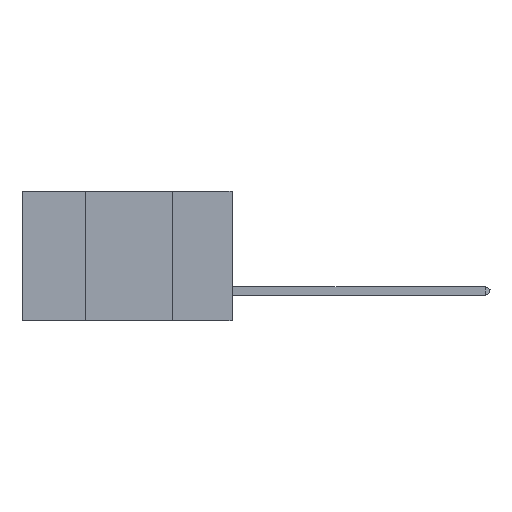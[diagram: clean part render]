
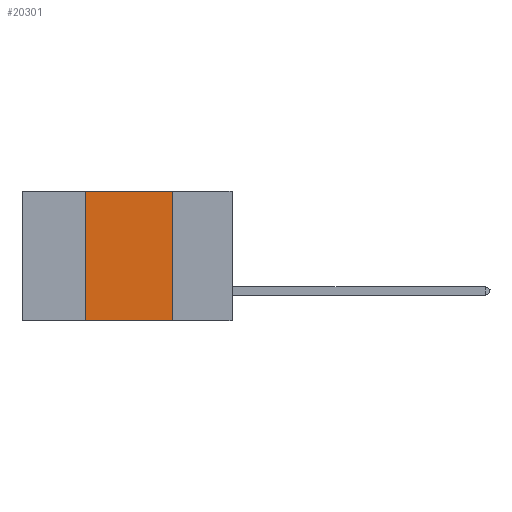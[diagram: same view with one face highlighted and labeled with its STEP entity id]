
A CAD part, left-side view. The second image highlights one B-rep face of the part: STEP entity #20301.
In plain terms, the highlighted planar face has unit normal (-1, 0, 0).
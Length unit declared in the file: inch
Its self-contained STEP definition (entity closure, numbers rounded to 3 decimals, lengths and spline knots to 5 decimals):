
#826 = VERTEX_POINT ( 'NONE', #9016 ) ;
#1259 = DIRECTION ( 'NONE',  ( 0., -1., 0. ) ) ;
#1552 = VECTOR ( 'NONE', #9663, 39.37008 ) ;
#1817 = LINE ( 'NONE', #21628, #24952 ) ;
#1890 = DIRECTION ( 'NONE',  ( 1., 0., 0. ) ) ;
#2437 = EDGE_CURVE ( 'NONE', #2929, #826, #20602, .T. ) ;
#2929 = VERTEX_POINT ( 'NONE', #21281 ) ;
#3544 = CARTESIAN_POINT ( 'NONE',  ( 0., 0.17, 0. ) ) ;
#6623 = VECTOR ( 'NONE', #12929, 39.37008 ) ;
#8155 = CARTESIAN_POINT ( 'NONE',  ( 0., 0.42, 0. ) ) ;
#8609 = VECTOR ( 'NONE', #1259, 39.37008 ) ;
#9016 = CARTESIAN_POINT ( 'NONE',  ( 0., 0.17, -0.37 ) ) ;
#9549 = ORIENTED_EDGE ( 'NONE', *, *, #26657, .F. ) ;
#9663 = DIRECTION ( 'NONE',  ( 0., 0., -1. ) ) ;
#9791 = CARTESIAN_POINT ( 'NONE',  ( 0., 0.6, -0.37 ) ) ;
#10098 = EDGE_LOOP ( 'NONE', ( #14602, #9549, #12467, #15605 ) ) ;
#10427 = PLANE ( 'NONE',  #12560 ) ;
#12229 = EDGE_CURVE ( 'NONE', #27784, #826, #15951, .T. ) ;
#12467 = ORIENTED_EDGE ( 'NONE', *, *, #16644, .F. ) ;
#12560 = AXIS2_PLACEMENT_3D ( 'NONE', #27599, #1890, #23340 ) ;
#12929 = DIRECTION ( 'NONE',  ( 0., 0., 1. ) ) ;
#13300 = VERTEX_POINT ( 'NONE', #8155 ) ;
#13327 = LINE ( 'NONE', #25845, #6623 ) ;
#14602 = ORIENTED_EDGE ( 'NONE', *, *, #12229, .F. ) ;
#15605 = ORIENTED_EDGE ( 'NONE', *, *, #2437, .T. ) ;
#15951 = LINE ( 'NONE', #3544, #1552 ) ;
#16644 = EDGE_CURVE ( 'NONE', #2929, #13300, #13327, .T. ) ;
#18490 = FACE_OUTER_BOUND ( 'NONE', #10098, .T. ) ;
#20301 = ADVANCED_FACE ( 'NONE', ( #18490 ), #10427, .F. ) ;
#20602 = LINE ( 'NONE', #9791, #8609 ) ;
#21281 = CARTESIAN_POINT ( 'NONE',  ( 0., 0.42, -0.37 ) ) ;
#21628 = CARTESIAN_POINT ( 'NONE',  ( 0., 0.6, 0. ) ) ;
#23340 = DIRECTION ( 'NONE',  ( 0., 0., -1. ) ) ;
#24952 = VECTOR ( 'NONE', #26086, 39.37008 ) ;
#25845 = CARTESIAN_POINT ( 'NONE',  ( 0., 0.42, 0. ) ) ;
#26086 = DIRECTION ( 'NONE',  ( 0., -1., 0. ) ) ;
#26657 = EDGE_CURVE ( 'NONE', #13300, #27784, #1817, .T. ) ;
#26976 = CARTESIAN_POINT ( 'NONE',  ( 0., 0.17, 0. ) ) ;
#27599 = CARTESIAN_POINT ( 'NONE',  ( 0., 0.6, 0. ) ) ;
#27784 = VERTEX_POINT ( 'NONE', #26976 ) ;
